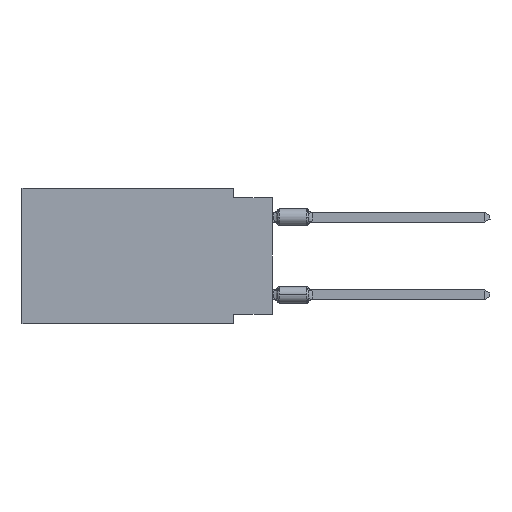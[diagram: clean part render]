
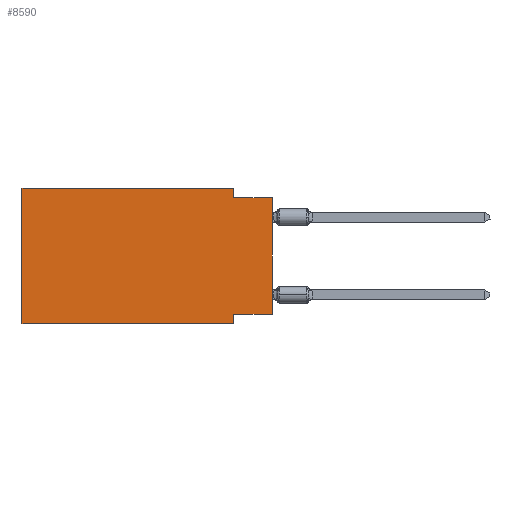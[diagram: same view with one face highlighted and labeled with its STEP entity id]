
A CAD part, left-side view. The second image highlights one B-rep face of the part: STEP entity #8590.
In plain terms, the highlighted planar face has unit normal (-1, 0, 0).
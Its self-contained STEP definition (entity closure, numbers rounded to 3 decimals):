
#197 = CARTESIAN_POINT ( 'NONE',  ( 0., 16.383, -8.89 ) ) ;
#742 = DIRECTION ( 'NONE',  ( 0., 0., -1. ) ) ;
#1416 = CARTESIAN_POINT ( 'NONE',  ( 0., 16.383, -8.89 ) ) ;
#2051 = CARTESIAN_POINT ( 'NONE',  ( 0., 2.54, 0. ) ) ;
#3383 = VERTEX_POINT ( 'NONE', #34431 ) ;
#4287 = DIRECTION ( 'NONE',  ( 0., -1., 0. ) ) ;
#4574 = LINE ( 'NONE', #10872, #11365 ) ;
#4621 = CARTESIAN_POINT ( 'NONE',  ( 0., 2.54, 0. ) ) ;
#4983 = DIRECTION ( 'NONE',  ( 0., 0., -1. ) ) ;
#5600 = VERTEX_POINT ( 'NONE', #18004 ) ;
#6288 = CARTESIAN_POINT ( 'NONE',  ( 0., 2.54, -8.89 ) ) ;
#8590 = ADVANCED_FACE ( 'NONE', ( #30838 ), #27576, .F. ) ;
#8665 = EDGE_CURVE ( 'NONE', #3383, #26439, #38637, .T. ) ;
#8900 = DIRECTION ( 'NONE',  ( 0., -1., 0. ) ) ;
#9043 = EDGE_CURVE ( 'NONE', #5600, #16426, #42256, .T. ) ;
#9947 = CARTESIAN_POINT ( 'NONE',  ( 0., 0., 0. ) ) ;
#9986 = ORIENTED_EDGE ( 'NONE', *, *, #9043, .F. ) ;
#10872 = CARTESIAN_POINT ( 'NONE',  ( 0., 2.54, -8.89 ) ) ;
#11365 = VECTOR ( 'NONE', #17813, 1000. ) ;
#12273 = EDGE_LOOP ( 'NONE', ( #31197, #16555, #13679, #14368, #13672, #41027, #32421, #9986 ) ) ;
#12587 = VECTOR ( 'NONE', #36192, 1000. ) ;
#13276 = VERTEX_POINT ( 'NONE', #1416 ) ;
#13672 = ORIENTED_EDGE ( 'NONE', *, *, #39582, .F. ) ;
#13679 = ORIENTED_EDGE ( 'NONE', *, *, #34371, .F. ) ;
#14368 = ORIENTED_EDGE ( 'NONE', *, *, #8665, .F. ) ;
#16039 = EDGE_CURVE ( 'NONE', #42584, #26331, #29697, .T. ) ;
#16426 = VERTEX_POINT ( 'NONE', #40952 ) ;
#16555 = ORIENTED_EDGE ( 'NONE', *, *, #16039, .F. ) ;
#17300 = VECTOR ( 'NONE', #35178, 1000. ) ;
#17813 = DIRECTION ( 'NONE',  ( 0., 0., -1. ) ) ;
#18004 = CARTESIAN_POINT ( 'NONE',  ( 0., 0., -8.255 ) ) ;
#19882 = VECTOR ( 'NONE', #4287, 1000. ) ;
#20155 = DIRECTION ( 'NONE',  ( 0., 0., 1. ) ) ;
#20932 = CARTESIAN_POINT ( 'NONE',  ( 0., 0., -0.635 ) ) ;
#21617 = EDGE_CURVE ( 'NONE', #13276, #29838, #23628, .T. ) ;
#22756 = CARTESIAN_POINT ( 'NONE',  ( 0., 0., -0.635 ) ) ;
#22777 = LINE ( 'NONE', #9947, #39372 ) ;
#23628 = LINE ( 'NONE', #197, #19882 ) ;
#25922 = VECTOR ( 'NONE', #8900, 1000. ) ;
#26331 = VERTEX_POINT ( 'NONE', #20932 ) ;
#26439 = VERTEX_POINT ( 'NONE', #2051 ) ;
#27576 = PLANE ( 'NONE',  #38398 ) ;
#29244 = DIRECTION ( 'NONE',  ( 0., 1., 0. ) ) ;
#29540 = EDGE_CURVE ( 'NONE', #16426, #29838, #4574, .T. ) ;
#29697 = LINE ( 'NONE', #22756, #12587 ) ;
#29838 = VERTEX_POINT ( 'NONE', #6288 ) ;
#30279 = VECTOR ( 'NONE', #742, 1000. ) ;
#30477 = LINE ( 'NONE', #4621, #30279 ) ;
#30764 = CARTESIAN_POINT ( 'NONE',  ( 0., 2.54, -0.635 ) ) ;
#30838 = FACE_OUTER_BOUND ( 'NONE', #12273, .T. ) ;
#31047 = CARTESIAN_POINT ( 'NONE',  ( 0., 16.383, 0. ) ) ;
#31197 = ORIENTED_EDGE ( 'NONE', *, *, #36711, .T. ) ;
#32421 = ORIENTED_EDGE ( 'NONE', *, *, #29540, .F. ) ;
#32515 = CARTESIAN_POINT ( 'NONE',  ( 0., 0., -8.255 ) ) ;
#34371 = EDGE_CURVE ( 'NONE', #26439, #42584, #30477, .T. ) ;
#34431 = CARTESIAN_POINT ( 'NONE',  ( 0., 16.383, 0. ) ) ;
#35178 = DIRECTION ( 'NONE',  ( 0., 0., 1. ) ) ;
#36192 = DIRECTION ( 'NONE',  ( 0., -1., 0. ) ) ;
#36711 = EDGE_CURVE ( 'NONE', #5600, #26331, #22777, .T. ) ;
#37986 = CARTESIAN_POINT ( 'NONE',  ( 0., 16.383, 0. ) ) ;
#38398 = AXIS2_PLACEMENT_3D ( 'NONE', #31047, #40801, #4983 ) ;
#38430 = VECTOR ( 'NONE', #29244, 1000. ) ;
#38637 = LINE ( 'NONE', #42098, #25922 ) ;
#39372 = VECTOR ( 'NONE', #20155, 1000. ) ;
#39582 = EDGE_CURVE ( 'NONE', #13276, #3383, #41447, .T. ) ;
#40801 = DIRECTION ( 'NONE',  ( 1., 0., 0. ) ) ;
#40952 = CARTESIAN_POINT ( 'NONE',  ( 0., 2.54, -8.255 ) ) ;
#41027 = ORIENTED_EDGE ( 'NONE', *, *, #21617, .T. ) ;
#41447 = LINE ( 'NONE', #37986, #17300 ) ;
#42098 = CARTESIAN_POINT ( 'NONE',  ( 0., 16.383, 0. ) ) ;
#42256 = LINE ( 'NONE', #32515, #38430 ) ;
#42584 = VERTEX_POINT ( 'NONE', #30764 ) ;
